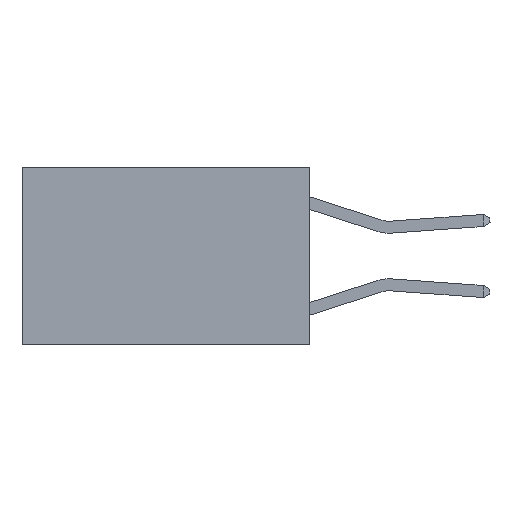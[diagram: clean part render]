
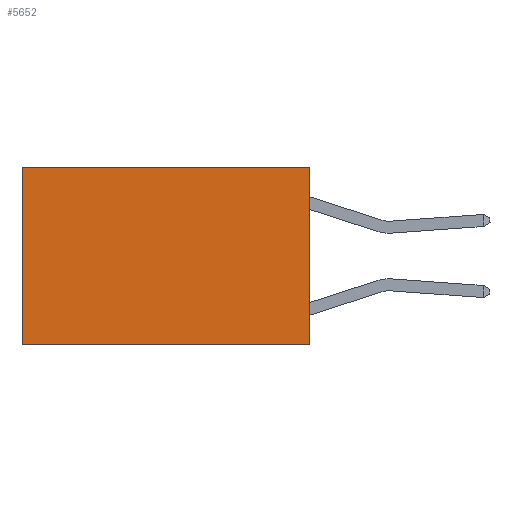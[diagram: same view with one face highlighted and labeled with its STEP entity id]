
A CAD part, left-side view. The second image highlights one B-rep face of the part: STEP entity #5652.
In plain terms, the highlighted planar face has unit normal (-1, 0, 0).
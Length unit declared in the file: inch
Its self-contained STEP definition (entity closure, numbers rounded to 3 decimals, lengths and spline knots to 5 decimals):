
#127 = VERTEX_POINT ( 'NONE', #7738 ) ;
#231 = DIRECTION ( 'NONE',  ( 0., 0., -1. ) ) ;
#454 = FACE_OUTER_BOUND ( 'NONE', #7011, .T. ) ;
#505 = LINE ( 'NONE', #5546, #6075 ) ;
#550 = EDGE_CURVE ( 'NONE', #2887, #6150, #4900, .T. ) ;
#634 = ORIENTED_EDGE ( 'NONE', *, *, #6309, .T. ) ;
#1559 = PLANE ( 'NONE',  #1703 ) ;
#1703 = AXIS2_PLACEMENT_3D ( 'NONE', #2320, #4827, #7353 ) ;
#1798 = CARTESIAN_POINT ( 'NONE',  ( 0.2625, 0., 0. ) ) ;
#2000 = EDGE_CURVE ( 'NONE', #4430, #127, #5761, .T. ) ;
#2137 = CARTESIAN_POINT ( 'NONE',  ( 0.2625, 0.6, 0. ) ) ;
#2320 = CARTESIAN_POINT ( 'NONE',  ( 0.2625, 0., 0. ) ) ;
#2639 = ORIENTED_EDGE ( 'NONE', *, *, #6511, .F. ) ;
#2887 = VERTEX_POINT ( 'NONE', #2137 ) ;
#3011 = CARTESIAN_POINT ( 'NONE',  ( 0.2625, 0.6, -0.37 ) ) ;
#3052 = VECTOR ( 'NONE', #4593, 39.37008 ) ;
#3058 = CARTESIAN_POINT ( 'NONE',  ( 0.2625, 0.6, 0. ) ) ;
#3312 = VECTOR ( 'NONE', #7341, 39.37008 ) ;
#3586 = ORIENTED_EDGE ( 'NONE', *, *, #550, .T. ) ;
#3907 = CARTESIAN_POINT ( 'NONE',  ( 0.2625, 0., 0. ) ) ;
#4388 = DIRECTION ( 'NONE',  ( 0., 1., 0. ) ) ;
#4430 = VERTEX_POINT ( 'NONE', #1798 ) ;
#4593 = DIRECTION ( 'NONE',  ( 0., 1., 0. ) ) ;
#4637 = CARTESIAN_POINT ( 'NONE',  ( 0.2625, 0., 0. ) ) ;
#4827 = DIRECTION ( 'NONE',  ( 1., 0., 0. ) ) ;
#4900 = LINE ( 'NONE', #3058, #3312 ) ;
#5546 = CARTESIAN_POINT ( 'NONE',  ( 0.2625, 0., -0.37 ) ) ;
#5652 = ADVANCED_FACE ( 'NONE', ( #454 ), #1559, .F. ) ;
#5761 = LINE ( 'NONE', #4637, #5963 ) ;
#5963 = VECTOR ( 'NONE', #231, 39.37008 ) ;
#6075 = VECTOR ( 'NONE', #4388, 39.37008 ) ;
#6150 = VERTEX_POINT ( 'NONE', #3011 ) ;
#6309 = EDGE_CURVE ( 'NONE', #4430, #2887, #7653, .T. ) ;
#6511 = EDGE_CURVE ( 'NONE', #127, #6150, #505, .T. ) ;
#7011 = EDGE_LOOP ( 'NONE', ( #3586, #2639, #8030, #634 ) ) ;
#7341 = DIRECTION ( 'NONE',  ( 0., 0., -1. ) ) ;
#7353 = DIRECTION ( 'NONE',  ( 0., 0., -1. ) ) ;
#7653 = LINE ( 'NONE', #3907, #3052 ) ;
#7738 = CARTESIAN_POINT ( 'NONE',  ( 0.2625, 0., -0.37 ) ) ;
#8030 = ORIENTED_EDGE ( 'NONE', *, *, #2000, .F. ) ;
